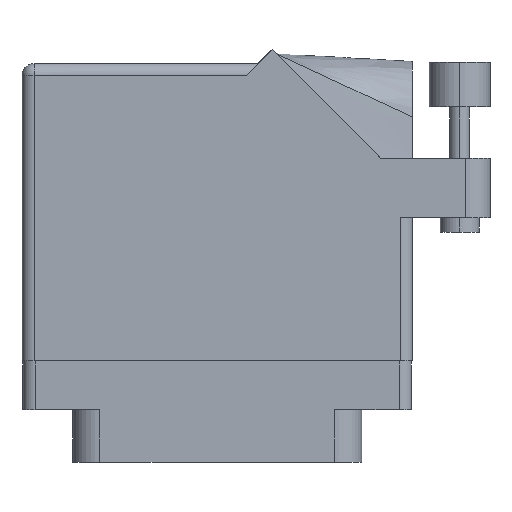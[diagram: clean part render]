
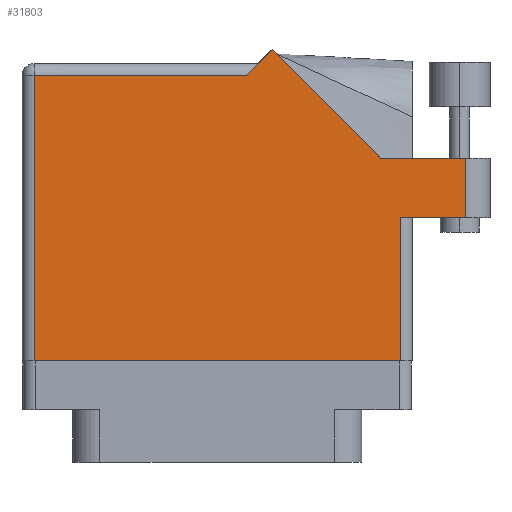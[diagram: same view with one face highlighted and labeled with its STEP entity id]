
A CAD part, front view. The second image highlights one B-rep face of the part: STEP entity #31803.
In plain terms, the highlighted face is planar.
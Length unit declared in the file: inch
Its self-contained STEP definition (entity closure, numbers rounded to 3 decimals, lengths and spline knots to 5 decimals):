
#206 = DIRECTION ( 'NONE',  ( 0., -1., 0. ) ) ;
#459 = CARTESIAN_POINT ( 'NONE',  ( -0.943, -0.1, 0.455 ) ) ;
#1394 = DIRECTION ( 'NONE',  ( -1., 0., 0. ) ) ;
#1767 = FACE_OUTER_BOUND ( 'NONE', #16466, .T. ) ;
#1812 = VERTEX_POINT ( 'NONE', #2460 ) ;
#2333 = LINE ( 'NONE', #37026, #23667 ) ;
#2460 = CARTESIAN_POINT ( 'NONE',  ( 0.15, 1.368, 0.455 ) ) ;
#2905 = ORIENTED_EDGE ( 'NONE', *, *, #12801, .T. ) ;
#2973 = LINE ( 'NONE', #11149, #26213 ) ;
#3282 = CARTESIAN_POINT ( 'NONE',  ( 0.943, -0.1, 0.455 ) ) ;
#4566 = ORIENTED_EDGE ( 'NONE', *, *, #17563, .T. ) ;
#4572 = CARTESIAN_POINT ( 'NONE',  ( -0.943, -0.1, 0.455 ) ) ;
#4691 = ORIENTED_EDGE ( 'NONE', *, *, #7848, .T. ) ;
#5227 = EDGE_CURVE ( 'NONE', #24345, #19227, #25430, .T. ) ;
#5799 = ORIENTED_EDGE ( 'NONE', *, *, #38837, .T. ) ;
#7374 = VERTEX_POINT ( 'NONE', #30859 ) ;
#7848 = EDGE_CURVE ( 'NONE', #12805, #24345, #11692, .T. ) ;
#9771 = CARTESIAN_POINT ( 'NONE',  ( 0.943, 0.637, 0.455 ) ) ;
#9934 = EDGE_CURVE ( 'NONE', #19227, #15003, #38402, .T. ) ;
#11149 = CARTESIAN_POINT ( 'NONE',  ( 0.83942, 0.944, 0.455 ) ) ;
#11214 = LINE ( 'NONE', #35297, #26692 ) ;
#11254 = CARTESIAN_POINT ( 'NONE',  ( 1.005, 0.637, 0.455 ) ) ;
#11328 = CARTESIAN_POINT ( 'NONE',  ( -1.005, 1.43, 0.455 ) ) ;
#11534 = AXIS2_PLACEMENT_3D ( 'NONE', #11328, #20653, #20911 ) ;
#11692 = LINE ( 'NONE', #459, #23292 ) ;
#12801 = EDGE_CURVE ( 'NONE', #17715, #1812, #2333, .T. ) ;
#12805 = VERTEX_POINT ( 'NONE', #32008 ) ;
#14420 = ORIENTED_EDGE ( 'NONE', *, *, #9934, .T. ) ;
#15003 = VERTEX_POINT ( 'NONE', #17248 ) ;
#16166 = VECTOR ( 'NONE', #19060, 39.37008 ) ;
#16466 = EDGE_LOOP ( 'NONE', ( #21606, #5799, #4566, #39145, #2905, #21063, #4691, #22714, #14420 ) ) ;
#16505 = VECTOR ( 'NONE', #37719, 39.37008 ) ;
#16861 = VECTOR ( 'NONE', #1394, 39.37008 ) ;
#17002 = LINE ( 'NONE', #11254, #16505 ) ;
#17248 = CARTESIAN_POINT ( 'NONE',  ( 0.943, 0.637, 0.455 ) ) ;
#17287 = VECTOR ( 'NONE', #32130, 39.37008 ) ;
#17563 = EDGE_CURVE ( 'NONE', #30265, #34452, #37171, .T. ) ;
#17715 = VERTEX_POINT ( 'NONE', #20317 ) ;
#19060 = DIRECTION ( 'NONE',  ( 0., 1., 0. ) ) ;
#19227 = VERTEX_POINT ( 'NONE', #3282 ) ;
#19329 = DIRECTION ( 'NONE',  ( 0., 1., 0. ) ) ;
#20317 = CARTESIAN_POINT ( 'NONE',  ( 0.28271, 1.50071, 0.455 ) ) ;
#20653 = DIRECTION ( 'NONE',  ( 0., 0., -1. ) ) ;
#20911 = DIRECTION ( 'NONE',  ( -1., 0., 0. ) ) ;
#21063 = ORIENTED_EDGE ( 'NONE', *, *, #25595, .T. ) ;
#21606 = ORIENTED_EDGE ( 'NONE', *, *, #38617, .T. ) ;
#22714 = ORIENTED_EDGE ( 'NONE', *, *, #5227, .T. ) ;
#23292 = VECTOR ( 'NONE', #206, 39.37008 ) ;
#23667 = VECTOR ( 'NONE', #34039, 39.37008 ) ;
#23749 = EDGE_CURVE ( 'NONE', #34452, #17715, #2973, .T. ) ;
#24345 = VERTEX_POINT ( 'NONE', #4572 ) ;
#25430 = LINE ( 'NONE', #30393, #31286 ) ;
#25595 = EDGE_CURVE ( 'NONE', #1812, #12805, #29483, .T. ) ;
#26213 = VECTOR ( 'NONE', #33073, 39.37008 ) ;
#26692 = VECTOR ( 'NONE', #19329, 39.37008 ) ;
#29483 = LINE ( 'NONE', #32526, #16861 ) ;
#30113 = DIRECTION ( 'NONE',  ( 1., 0., 0. ) ) ;
#30265 = VERTEX_POINT ( 'NONE', #33758 ) ;
#30393 = CARTESIAN_POINT ( 'NONE',  ( -1.005, -0.1, 0.455 ) ) ;
#30859 = CARTESIAN_POINT ( 'NONE',  ( 1.28, 0.637, 0.455 ) ) ;
#31286 = VECTOR ( 'NONE', #30113, 39.37008 ) ;
#31803 = ADVANCED_FACE ( 'NONE', ( #1767 ), #36210, .F. ) ;
#32008 = CARTESIAN_POINT ( 'NONE',  ( -0.943, 1.368, 0.455 ) ) ;
#32130 = DIRECTION ( 'NONE',  ( -1., 0., 0. ) ) ;
#32526 = CARTESIAN_POINT ( 'NONE',  ( -1.005, 1.368, 0.455 ) ) ;
#33073 = DIRECTION ( 'NONE',  ( -0.707, 0.707, 0. ) ) ;
#33758 = CARTESIAN_POINT ( 'NONE',  ( 1.28, 0.944, 0.455 ) ) ;
#34039 = DIRECTION ( 'NONE',  ( -0.707, -0.707, 0. ) ) ;
#34452 = VERTEX_POINT ( 'NONE', #37472 ) ;
#35297 = CARTESIAN_POINT ( 'NONE',  ( 1.28, 0.944, 0.455 ) ) ;
#36210 = PLANE ( 'NONE',  #11534 ) ;
#37026 = CARTESIAN_POINT ( 'NONE',  ( 0.212, 1.43, 0.455 ) ) ;
#37171 = LINE ( 'NONE', #38686, #17287 ) ;
#37472 = CARTESIAN_POINT ( 'NONE',  ( 0.83942, 0.944, 0.455 ) ) ;
#37719 = DIRECTION ( 'NONE',  ( 1., 0., 0. ) ) ;
#38402 = LINE ( 'NONE', #9771, #16166 ) ;
#38617 = EDGE_CURVE ( 'NONE', #15003, #7374, #17002, .T. ) ;
#38686 = CARTESIAN_POINT ( 'NONE',  ( 1.405, 0.944, 0.455 ) ) ;
#38837 = EDGE_CURVE ( 'NONE', #7374, #30265, #11214, .T. ) ;
#39145 = ORIENTED_EDGE ( 'NONE', *, *, #23749, .T. ) ;
